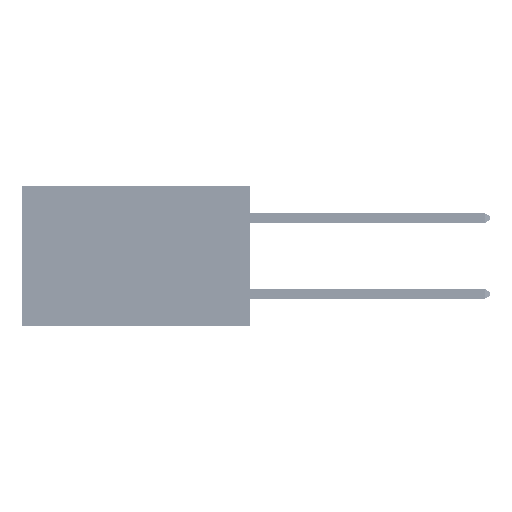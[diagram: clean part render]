
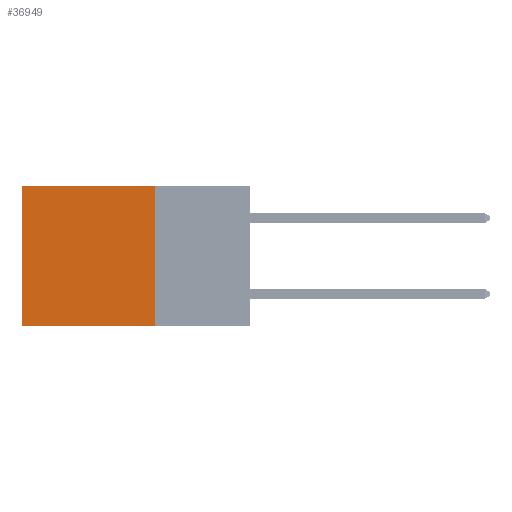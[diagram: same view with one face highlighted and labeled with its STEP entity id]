
A CAD part, left-side view. The second image highlights one B-rep face of the part: STEP entity #36949.
In plain terms, the highlighted planar face has unit normal (-1, 0, 0).
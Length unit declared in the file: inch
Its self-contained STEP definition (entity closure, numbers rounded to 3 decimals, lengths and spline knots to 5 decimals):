
#1006 = ORIENTED_EDGE ( 'NONE', *, *, #35779, .F. ) ;
#2557 = LINE ( 'NONE', #7329, #27505 ) ;
#3409 = CARTESIAN_POINT ( 'NONE',  ( 0.2875, 0.6, -0.37 ) ) ;
#5103 = ORIENTED_EDGE ( 'NONE', *, *, #39566, .T. ) ;
#6248 = VERTEX_POINT ( 'NONE', #29285 ) ;
#6373 = CARTESIAN_POINT ( 'NONE',  ( 0.2875, 0.6, 0. ) ) ;
#7329 = CARTESIAN_POINT ( 'NONE',  ( 0.2875, 0.6, 0. ) ) ;
#9640 = EDGE_LOOP ( 'NONE', ( #5103, #1006, #22775, #49485 ) ) ;
#12119 = EDGE_CURVE ( 'NONE', #39434, #6248, #23749, .T. ) ;
#13141 = VERTEX_POINT ( 'NONE', #6373 ) ;
#17405 = CARTESIAN_POINT ( 'NONE',  ( 0.2875, 0.25, 0. ) ) ;
#17591 = CARTESIAN_POINT ( 'NONE',  ( 0.2875, 0.25, 0. ) ) ;
#18692 = LINE ( 'NONE', #50710, #28180 ) ;
#19686 = PLANE ( 'NONE',  #26584 ) ;
#20823 = VECTOR ( 'NONE', #48345, 39.37008 ) ;
#22775 = ORIENTED_EDGE ( 'NONE', *, *, #12119, .F. ) ;
#23479 = DIRECTION ( 'NONE',  ( 0., 0., -1. ) ) ;
#23663 = FACE_OUTER_BOUND ( 'NONE', #9640, .T. ) ;
#23749 = LINE ( 'NONE', #43624, #20823 ) ;
#26584 = AXIS2_PLACEMENT_3D ( 'NONE', #39818, #27115, #51711 ) ;
#27115 = DIRECTION ( 'NONE',  ( 1., 0., 0. ) ) ;
#27325 = VERTEX_POINT ( 'NONE', #3409 ) ;
#27505 = VECTOR ( 'NONE', #23479, 39.37008 ) ;
#28180 = VECTOR ( 'NONE', #38306, 39.37008 ) ;
#29285 = CARTESIAN_POINT ( 'NONE',  ( 0.2875, 0.25, -0.37 ) ) ;
#29945 = VECTOR ( 'NONE', #41965, 39.37008 ) ;
#35779 = EDGE_CURVE ( 'NONE', #6248, #27325, #18692, .T. ) ;
#36857 = EDGE_CURVE ( 'NONE', #39434, #13141, #37024, .T. ) ;
#36949 = ADVANCED_FACE ( 'NONE', ( #23663 ), #19686, .F. ) ;
#37024 = LINE ( 'NONE', #17591, #29945 ) ;
#38306 = DIRECTION ( 'NONE',  ( 0., 1., 0. ) ) ;
#39434 = VERTEX_POINT ( 'NONE', #17405 ) ;
#39566 = EDGE_CURVE ( 'NONE', #13141, #27325, #2557, .T. ) ;
#39818 = CARTESIAN_POINT ( 'NONE',  ( 0.2875, 0.25, 0. ) ) ;
#41965 = DIRECTION ( 'NONE',  ( 0., 1., 0. ) ) ;
#43624 = CARTESIAN_POINT ( 'NONE',  ( 0.2875, 0.25, 0. ) ) ;
#48345 = DIRECTION ( 'NONE',  ( 0., 0., -1. ) ) ;
#49485 = ORIENTED_EDGE ( 'NONE', *, *, #36857, .T. ) ;
#50710 = CARTESIAN_POINT ( 'NONE',  ( 0.2875, 0.25, -0.37 ) ) ;
#51711 = DIRECTION ( 'NONE',  ( 0., 0., -1. ) ) ;
